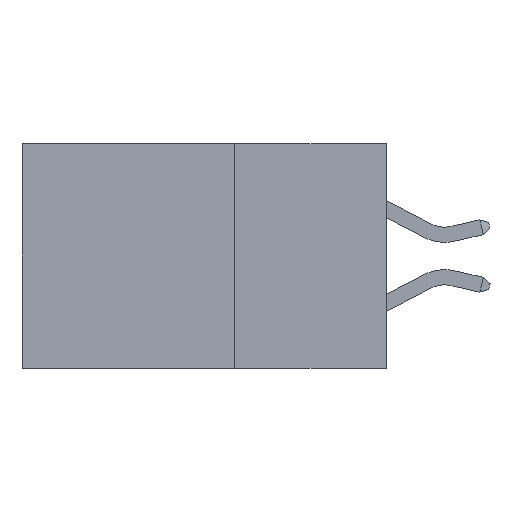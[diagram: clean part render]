
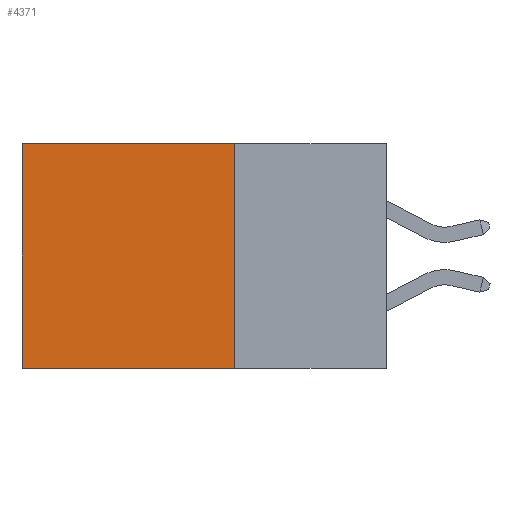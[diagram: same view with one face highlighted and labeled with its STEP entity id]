
A CAD part, left-side view. The second image highlights one B-rep face of the part: STEP entity #4371.
In plain terms, the highlighted planar face has unit normal (-1, 0, 0).
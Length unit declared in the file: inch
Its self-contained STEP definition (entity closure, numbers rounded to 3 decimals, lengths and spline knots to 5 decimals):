
#365 = CARTESIAN_POINT ( 'NONE',  ( 0.298, 0.6, 0. ) ) ;
#500 = EDGE_CURVE ( 'NONE', #2656, #3199, #4934, .T. ) ;
#1551 = ORIENTED_EDGE ( 'NONE', *, *, #10585, .F. ) ;
#1626 = CARTESIAN_POINT ( 'NONE',  ( 0.298, 0.25, -0.37 ) ) ;
#1799 = VECTOR ( 'NONE', #2680, 39.37008 ) ;
#2656 = VERTEX_POINT ( 'NONE', #10814 ) ;
#2680 = DIRECTION ( 'NONE',  ( 0., 0., -1. ) ) ;
#2867 = DIRECTION ( 'NONE',  ( 0., 1., 0. ) ) ;
#3199 = VERTEX_POINT ( 'NONE', #365 ) ;
#3521 = VECTOR ( 'NONE', #10621, 39.37008 ) ;
#4014 = VERTEX_POINT ( 'NONE', #4857 ) ;
#4179 = EDGE_CURVE ( 'NONE', #2656, #5987, #11670, .T. ) ;
#4371 = ADVANCED_FACE ( 'NONE', ( #4558 ), #8048, .F. ) ;
#4521 = AXIS2_PLACEMENT_3D ( 'NONE', #10097, #9964, #5334 ) ;
#4558 = FACE_OUTER_BOUND ( 'NONE', #6439, .T. ) ;
#4857 = CARTESIAN_POINT ( 'NONE',  ( 0.298, 0.6, -0.37 ) ) ;
#4934 = LINE ( 'NONE', #8510, #9419 ) ;
#5130 = EDGE_CURVE ( 'NONE', #3199, #4014, #6259, .T. ) ;
#5334 = DIRECTION ( 'NONE',  ( 0., 0., -1. ) ) ;
#5987 = VERTEX_POINT ( 'NONE', #8695 ) ;
#6209 = ORIENTED_EDGE ( 'NONE', *, *, #500, .T. ) ;
#6259 = LINE ( 'NONE', #8740, #3521 ) ;
#6264 = VECTOR ( 'NONE', #8962, 39.37008 ) ;
#6439 = EDGE_LOOP ( 'NONE', ( #6682, #1551, #8526, #6209 ) ) ;
#6682 = ORIENTED_EDGE ( 'NONE', *, *, #5130, .T. ) ;
#8048 = PLANE ( 'NONE',  #4521 ) ;
#8510 = CARTESIAN_POINT ( 'NONE',  ( 0.298, 0.25, 0. ) ) ;
#8526 = ORIENTED_EDGE ( 'NONE', *, *, #4179, .F. ) ;
#8695 = CARTESIAN_POINT ( 'NONE',  ( 0.298, 0.25, -0.37 ) ) ;
#8740 = CARTESIAN_POINT ( 'NONE',  ( 0.298, 0.6, 0. ) ) ;
#8747 = LINE ( 'NONE', #1626, #6264 ) ;
#8962 = DIRECTION ( 'NONE',  ( 0., 1., 0. ) ) ;
#9419 = VECTOR ( 'NONE', #2867, 39.37008 ) ;
#9964 = DIRECTION ( 'NONE',  ( 1., 0., 0. ) ) ;
#10097 = CARTESIAN_POINT ( 'NONE',  ( 0.298, 0.25, 0. ) ) ;
#10585 = EDGE_CURVE ( 'NONE', #5987, #4014, #8747, .T. ) ;
#10621 = DIRECTION ( 'NONE',  ( 0., 0., -1. ) ) ;
#10814 = CARTESIAN_POINT ( 'NONE',  ( 0.298, 0.25, 0. ) ) ;
#11670 = LINE ( 'NONE', #11671, #1799 ) ;
#11671 = CARTESIAN_POINT ( 'NONE',  ( 0.298, 0.25, 0. ) ) ;
